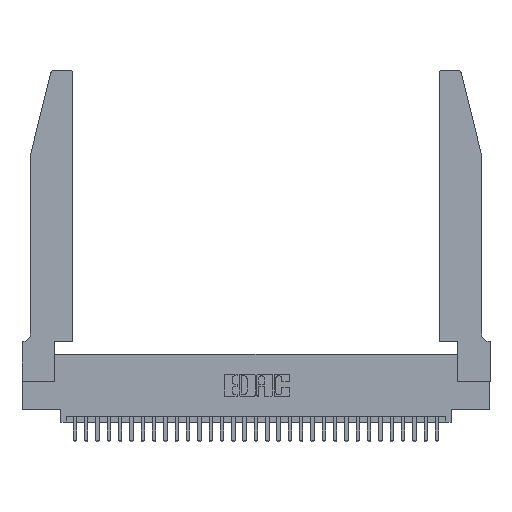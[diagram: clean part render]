
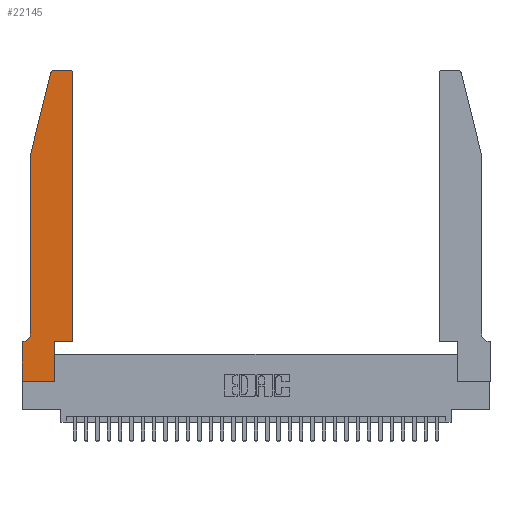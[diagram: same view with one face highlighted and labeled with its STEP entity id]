
A CAD part, top view. The second image highlights one B-rep face of the part: STEP entity #22145.
In plain terms, the highlighted planar face has unit normal (0, 0, 1).
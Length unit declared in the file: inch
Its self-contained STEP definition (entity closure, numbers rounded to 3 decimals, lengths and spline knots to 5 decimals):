
#126 = CARTESIAN_POINT ( 'NONE',  ( 0.4205, 2.72, 0.37 ) ) ;
#208 = ORIENTED_EDGE ( 'NONE', *, *, #18326, .T. ) ;
#269 = CARTESIAN_POINT ( 'NONE',  ( 0.0055, 0.35, 0.37 ) ) ;
#542 = LINE ( 'NONE', #15213, #26964 ) ;
#1882 = EDGE_CURVE ( 'NONE', #21220, #5612, #18966, .T. ) ;
#2193 = LINE ( 'NONE', #31049, #21141 ) ;
#2643 = DIRECTION ( 'NONE',  ( 1., 0., 0. ) ) ;
#2846 = DIRECTION ( 'NONE',  ( -1., 0., 0. ) ) ;
#2861 = DIRECTION ( 'NONE',  ( 1., 0., 0. ) ) ;
#3453 = VECTOR ( 'NONE', #11098, 39.37008 ) ;
#3671 = VERTEX_POINT ( 'NONE', #25404 ) ;
#4033 = CARTESIAN_POINT ( 'NONE',  ( 0.0755, 0.42, 0.37 ) ) ;
#4094 = AXIS2_PLACEMENT_3D ( 'NONE', #4150, #21403, #6639 ) ;
#4150 = CARTESIAN_POINT ( 'NONE',  ( 0.0055, 0.42, 0.37 ) ) ;
#4590 = CARTESIAN_POINT ( 'NONE',  ( 0.4505, 0.35, 0.37 ) ) ;
#4993 = CIRCLE ( 'NONE', #14402, 0.03 ) ;
#4996 = CARTESIAN_POINT ( 'NONE',  ( 0.2605, 2.75, 0.37 ) ) ;
#5127 = CARTESIAN_POINT ( 'NONE',  ( 0.0755, 2., 0.37 ) ) ;
#5192 = ORIENTED_EDGE ( 'NONE', *, *, #10550, .T. ) ;
#5399 = DIRECTION ( 'NONE',  ( 0., 1., 0. ) ) ;
#5612 = VERTEX_POINT ( 'NONE', #8401 ) ;
#5725 = VERTEX_POINT ( 'NONE', #4033 ) ;
#6028 = EDGE_CURVE ( 'NONE', #30564, #18628, #26151, .T. ) ;
#6285 = CARTESIAN_POINT ( 'NONE',  ( 0., 0.35, 0.37 ) ) ;
#6390 = DIRECTION ( 'NONE',  ( 0., -1., 0. ) ) ;
#6494 = ORIENTED_EDGE ( 'NONE', *, *, #23489, .T. ) ;
#6639 = DIRECTION ( 'NONE',  ( -1., 0., 0. ) ) ;
#6943 = AXIS2_PLACEMENT_3D ( 'NONE', #28905, #14053, #31364 ) ;
#7616 = DIRECTION ( 'NONE',  ( -0.239, -0.971, 0. ) ) ;
#7769 = EDGE_LOOP ( 'NONE', ( #11721, #6494, #208, #11991, #5192, #24463, #31918, #29866, #8741, #21261, #27744, #22041 ) ) ;
#8055 = CARTESIAN_POINT ( 'NONE',  ( 0.0755, 0.35, 0.37 ) ) ;
#8398 = LINE ( 'NONE', #25188, #20690 ) ;
#8401 = CARTESIAN_POINT ( 'NONE',  ( 0.284, 2.75, 0.37 ) ) ;
#8529 = VERTEX_POINT ( 'NONE', #10670 ) ;
#8741 = ORIENTED_EDGE ( 'NONE', *, *, #25600, .T. ) ;
#9621 = DIRECTION ( 'NONE',  ( 0., 0., 1. ) ) ;
#10066 = LINE ( 'NONE', #15937, #3453 ) ;
#10550 = EDGE_CURVE ( 'NONE', #5725, #30564, #22723, .T. ) ;
#10570 = CIRCLE ( 'NONE', #11575, 0.03 ) ;
#10670 = CARTESIAN_POINT ( 'NONE',  ( 0., 0., 0.37 ) ) ;
#11098 = DIRECTION ( 'NONE',  ( 0., 1., 0. ) ) ;
#11447 = LINE ( 'NONE', #4590, #30441 ) ;
#11575 = AXIS2_PLACEMENT_3D ( 'NONE', #126, #17479, #2643 ) ;
#11578 = PLANE ( 'NONE',  #6943 ) ;
#11721 = ORIENTED_EDGE ( 'NONE', *, *, #1882, .T. ) ;
#11991 = ORIENTED_EDGE ( 'NONE', *, *, #18648, .T. ) ;
#14053 = DIRECTION ( 'NONE',  ( 0., 0., 1. ) ) ;
#14266 = VECTOR ( 'NONE', #17334, 39.37008 ) ;
#14278 = VERTEX_POINT ( 'NONE', #23601 ) ;
#14402 = AXIS2_PLACEMENT_3D ( 'NONE', #24439, #9621, #26959 ) ;
#14857 = CARTESIAN_POINT ( 'NONE',  ( 0., 0., 0.37 ) ) ;
#15104 = EDGE_CURVE ( 'NONE', #29463, #21220, #10570, .T. ) ;
#15213 = CARTESIAN_POINT ( 'NONE',  ( 0., 0., 0.37 ) ) ;
#15470 = DIRECTION ( 'NONE',  ( -1., 0., 0. ) ) ;
#15589 = CARTESIAN_POINT ( 'NONE',  ( 0.4505, 0.35, 0.37 ) ) ;
#15937 = CARTESIAN_POINT ( 'NONE',  ( 0.4505, 0.35, 0.37 ) ) ;
#17322 = VECTOR ( 'NONE', #7616, 39.37008 ) ;
#17334 = DIRECTION ( 'NONE',  ( 0., -1., 0. ) ) ;
#17471 = EDGE_CURVE ( 'NONE', #24520, #29463, #10066, .T. ) ;
#17479 = DIRECTION ( 'NONE',  ( 0., 0., 1. ) ) ;
#18217 = VECTOR ( 'NONE', #2846, 39.37008 ) ;
#18326 = EDGE_CURVE ( 'NONE', #14278, #30916, #24724, .T. ) ;
#18628 = VERTEX_POINT ( 'NONE', #6285 ) ;
#18648 = EDGE_CURVE ( 'NONE', #30916, #5725, #2193, .T. ) ;
#18694 = VECTOR ( 'NONE', #15470, 39.37008 ) ;
#18966 = LINE ( 'NONE', #4996, #18217 ) ;
#19755 = EDGE_CURVE ( 'NONE', #3671, #24520, #11447, .T. ) ;
#20227 = CARTESIAN_POINT ( 'NONE',  ( 0.4205, 2.75, 0.37 ) ) ;
#20690 = VECTOR ( 'NONE', #5399, 39.37008 ) ;
#21141 = VECTOR ( 'NONE', #6390, 39.37008 ) ;
#21220 = VERTEX_POINT ( 'NONE', #20227 ) ;
#21261 = ORIENTED_EDGE ( 'NONE', *, *, #19755, .T. ) ;
#21403 = DIRECTION ( 'NONE',  ( 0., 0., -1. ) ) ;
#21832 = DIRECTION ( 'NONE',  ( 1., 0., 0. ) ) ;
#22041 = ORIENTED_EDGE ( 'NONE', *, *, #15104, .T. ) ;
#22145 = ADVANCED_FACE ( 'NONE', ( #22450 ), #11578, .T. ) ;
#22450 = FACE_OUTER_BOUND ( 'NONE', #7769, .T. ) ;
#22723 = CIRCLE ( 'NONE', #4094, 0.07 ) ;
#22886 = CARTESIAN_POINT ( 'NONE',  ( 0.4505, 2.72, 0.37 ) ) ;
#23094 = CARTESIAN_POINT ( 'NONE',  ( 0.2865, 0., 0.37 ) ) ;
#23489 = EDGE_CURVE ( 'NONE', #5612, #14278, #4993, .T. ) ;
#23601 = CARTESIAN_POINT ( 'NONE',  ( 0.25487, 2.72718, 0.37 ) ) ;
#24439 = CARTESIAN_POINT ( 'NONE',  ( 0.284, 2.72, 0.37 ) ) ;
#24463 = ORIENTED_EDGE ( 'NONE', *, *, #6028, .T. ) ;
#24520 = VERTEX_POINT ( 'NONE', #15589 ) ;
#24724 = LINE ( 'NONE', #5127, #17322 ) ;
#25188 = CARTESIAN_POINT ( 'NONE',  ( 0.2865, 0.35, 0.37 ) ) ;
#25404 = CARTESIAN_POINT ( 'NONE',  ( 0.2865, 0.35, 0.37 ) ) ;
#25600 = EDGE_CURVE ( 'NONE', #27740, #3671, #8398, .T. ) ;
#26151 = LINE ( 'NONE', #8055, #18694 ) ;
#26959 = DIRECTION ( 'NONE',  ( 1., 0., 0. ) ) ;
#26964 = VECTOR ( 'NONE', #2861, 39.37008 ) ;
#27491 = LINE ( 'NONE', #14857, #14266 ) ;
#27740 = VERTEX_POINT ( 'NONE', #23094 ) ;
#27744 = ORIENTED_EDGE ( 'NONE', *, *, #17471, .T. ) ;
#28905 = CARTESIAN_POINT ( 'NONE',  ( 0., 0.35, 0.37 ) ) ;
#29463 = VERTEX_POINT ( 'NONE', #22886 ) ;
#29866 = ORIENTED_EDGE ( 'NONE', *, *, #32087, .T. ) ;
#29949 = EDGE_CURVE ( 'NONE', #18628, #8529, #27491, .T. ) ;
#30441 = VECTOR ( 'NONE', #21832, 39.37008 ) ;
#30564 = VERTEX_POINT ( 'NONE', #269 ) ;
#30916 = VERTEX_POINT ( 'NONE', #31793 ) ;
#31049 = CARTESIAN_POINT ( 'NONE',  ( 0.0755, 2., 0.37 ) ) ;
#31364 = DIRECTION ( 'NONE',  ( 1., 0., 0. ) ) ;
#31793 = CARTESIAN_POINT ( 'NONE',  ( 0.0755, 2., 0.37 ) ) ;
#31918 = ORIENTED_EDGE ( 'NONE', *, *, #29949, .T. ) ;
#32087 = EDGE_CURVE ( 'NONE', #8529, #27740, #542, .T. ) ;
